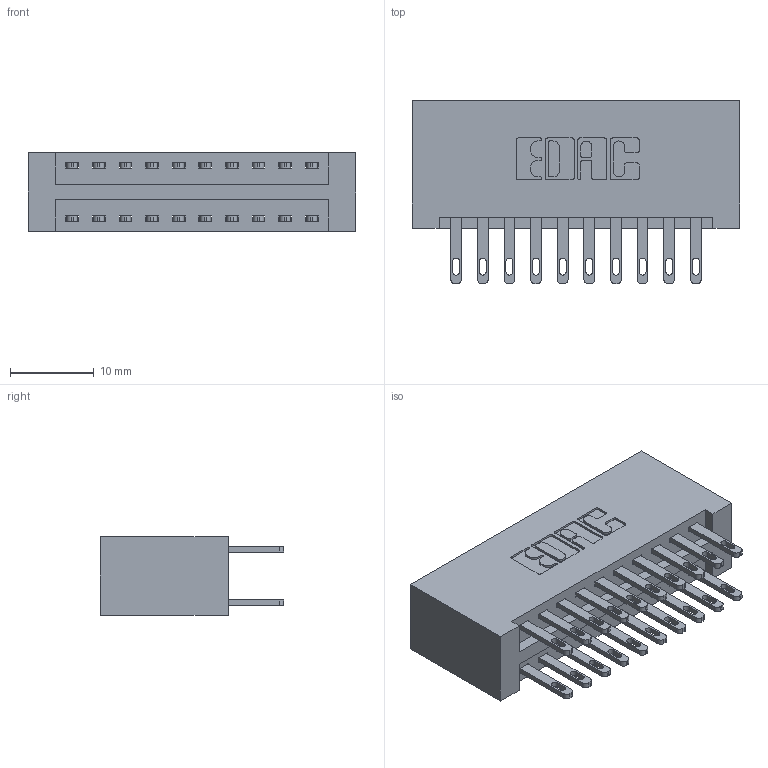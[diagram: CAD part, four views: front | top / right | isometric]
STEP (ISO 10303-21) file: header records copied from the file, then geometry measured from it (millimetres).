
FILE_DESCRIPTION (( 'STEP AP203' ), '1' );
FILE_NAME ('896-020-500-201.STEP', '2021-07-27T16:26:00', ( '' ), ( '' ), 'SwSTEP 2.0', 'SolidWorks 2020', '' );
FILE_SCHEMA (( 'CONFIG_CONTROL_DESIGN' ));
Length unit declared in the file: inch
Products named in the file (3): 846 Part_No Mounting Lugs; 896-020-500-201; 345-292-001_345-293-100
Assembly tree (21 placements, depth 2):
  896-020-500-201
    846 Part_No Mounting Lugs
    345-292-001_345-293-100  x20
Bounding box: 38.99 x 21.84 x 9.4 mm (x, y, z)
Volume: 4187.8 mm3; surface area: 5625.9 mm2
Topology: 21 solids, 21 shells, 1074 faces, 3245 edges, 2162 vertices
Faces by surface type: plane 652, cylinder 422
Entity records: 10487 total; most frequent: CARTESIAN_POINT 1768, ORIENTED_EDGE 1702, DIRECTION 1607, EDGE_CURVE 851, LINE 683, VECTOR 683, VERTEX_POINT 566, AXIS2_PLACEMENT_3D 462
